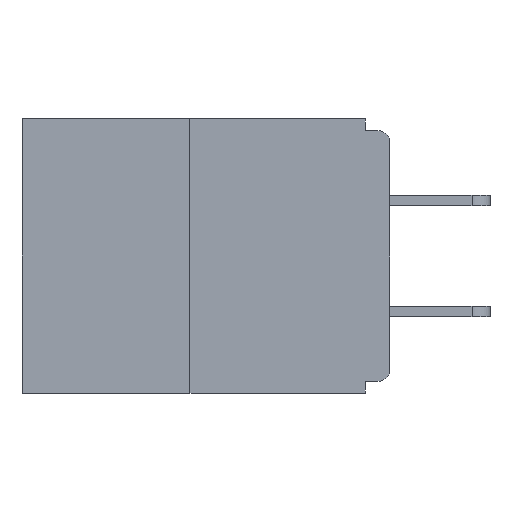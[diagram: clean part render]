
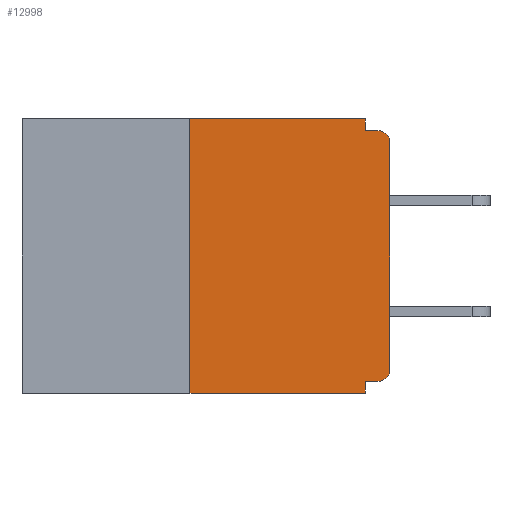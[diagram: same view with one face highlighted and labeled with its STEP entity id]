
A CAD part, left-side view. The second image highlights one B-rep face of the part: STEP entity #12998.
In plain terms, the highlighted planar face has unit normal (-1, 0, 0).
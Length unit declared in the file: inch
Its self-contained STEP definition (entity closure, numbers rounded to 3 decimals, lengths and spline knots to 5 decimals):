
#118 = DIRECTION ( 'NONE',  ( 0., 0., -1. ) ) ;
#300 = ORIENTED_EDGE ( 'NONE', *, *, #8440, .T. ) ;
#609 = VERTEX_POINT ( 'NONE', #5501 ) ;
#693 = CARTESIAN_POINT ( 'NONE',  ( 0., 0.015, -0.313 ) ) ;
#877 = DIRECTION ( 'NONE',  ( 0., -1., 0. ) ) ;
#916 = VECTOR ( 'NONE', #6796, 39.37008 ) ;
#1182 = DIRECTION ( 'NONE',  ( 0., 0., -1. ) ) ;
#2056 = LINE ( 'NONE', #11511, #4643 ) ;
#2653 = ORIENTED_EDGE ( 'NONE', *, *, #12278, .F. ) ;
#2808 = EDGE_CURVE ( 'NONE', #11994, #15550, #15641, .T. ) ;
#2951 = LINE ( 'NONE', #13225, #12132 ) ;
#3209 = CARTESIAN_POINT ( 'NONE',  ( 0., 0., -0.03 ) ) ;
#3536 = DIRECTION ( 'NONE',  ( 0., 0., 1. ) ) ;
#4190 = VERTEX_POINT ( 'NONE', #11120 ) ;
#4578 = EDGE_LOOP ( 'NONE', ( #9824, #7527, #5106, #11072, #5703, #300, #7327, #6595, #2653, #16163 ) ) ;
#4643 = VECTOR ( 'NONE', #1182, 39.37008 ) ;
#5106 = ORIENTED_EDGE ( 'NONE', *, *, #10989, .T. ) ;
#5346 = CARTESIAN_POINT ( 'NONE',  ( 0., 0., -0.015 ) ) ;
#5501 = CARTESIAN_POINT ( 'NONE',  ( 0., 0.015, -0.328 ) ) ;
#5656 = CARTESIAN_POINT ( 'NONE',  ( 0., 0.031, -0.328 ) ) ;
#5703 = ORIENTED_EDGE ( 'NONE', *, *, #7304, .F. ) ;
#5862 = CARTESIAN_POINT ( 'NONE',  ( 0., 0.031, -0.015 ) ) ;
#6021 = VERTEX_POINT ( 'NONE', #15294 ) ;
#6104 = VERTEX_POINT ( 'NONE', #5656 ) ;
#6595 = ORIENTED_EDGE ( 'NONE', *, *, #2808, .T. ) ;
#6708 = FACE_OUTER_BOUND ( 'NONE', #4578, .T. ) ;
#6796 = DIRECTION ( 'NONE',  ( 0., -1., 0. ) ) ;
#6824 = AXIS2_PLACEMENT_3D ( 'NONE', #693, #12034, #11977 ) ;
#6897 = CARTESIAN_POINT ( 'NONE',  ( 0., 0.015, -0.015 ) ) ;
#7217 = EDGE_CURVE ( 'NONE', #13805, #13820, #2056, .T. ) ;
#7221 = VECTOR ( 'NONE', #3536, 39.37008 ) ;
#7253 = CARTESIAN_POINT ( 'NONE',  ( 0., 0.46, 0. ) ) ;
#7304 = EDGE_CURVE ( 'NONE', #609, #6104, #11629, .T. ) ;
#7327 = ORIENTED_EDGE ( 'NONE', *, *, #16149, .T. ) ;
#7527 = ORIENTED_EDGE ( 'NONE', *, *, #11657, .F. ) ;
#7826 = VERTEX_POINT ( 'NONE', #14133 ) ;
#7867 = VECTOR ( 'NONE', #10351, 39.37008 ) ;
#8162 = LINE ( 'NONE', #11536, #14740 ) ;
#8440 = EDGE_CURVE ( 'NONE', #609, #4190, #14588, .T. ) ;
#9077 = CARTESIAN_POINT ( 'NONE',  ( 0., 0.015, -0.03 ) ) ;
#9128 = CARTESIAN_POINT ( 'NONE',  ( 0., 0., -0.328 ) ) ;
#9378 = LINE ( 'NONE', #7253, #15359 ) ;
#9507 = LINE ( 'NONE', #15644, #916 ) ;
#9747 = CARTESIAN_POINT ( 'NONE',  ( 0., 0.031, 0. ) ) ;
#9824 = ORIENTED_EDGE ( 'NONE', *, *, #9898, .F. ) ;
#9898 = EDGE_CURVE ( 'NONE', #14648, #13805, #9378, .T. ) ;
#10116 = VECTOR ( 'NONE', #14479, 39.37008 ) ;
#10157 = DIRECTION ( 'NONE',  ( 0., 0., 1. ) ) ;
#10245 = DIRECTION ( 'NONE',  ( -1., 0., 0. ) ) ;
#10293 = AXIS2_PLACEMENT_3D ( 'NONE', #9077, #10245, #118 ) ;
#10351 = DIRECTION ( 'NONE',  ( 0., 1., 0. ) ) ;
#10369 = EDGE_CURVE ( 'NONE', #6104, #7826, #2951, .T. ) ;
#10850 = DIRECTION ( 'NONE',  ( 0., 0., -1. ) ) ;
#10989 = EDGE_CURVE ( 'NONE', #6021, #7826, #9507, .T. ) ;
#11023 = CARTESIAN_POINT ( 'NONE',  ( 0., 0.46, 0. ) ) ;
#11072 = ORIENTED_EDGE ( 'NONE', *, *, #10369, .F. ) ;
#11120 = CARTESIAN_POINT ( 'NONE',  ( 0., 0., -0.313 ) ) ;
#11250 = CARTESIAN_POINT ( 'NONE',  ( 0., 0.25, 0. ) ) ;
#11511 = CARTESIAN_POINT ( 'NONE',  ( 0., 0.031, 0. ) ) ;
#11536 = CARTESIAN_POINT ( 'NONE',  ( 0., 0.25, 0. ) ) ;
#11629 = LINE ( 'NONE', #9128, #7867 ) ;
#11657 = EDGE_CURVE ( 'NONE', #6021, #14648, #8162, .T. ) ;
#11711 = CARTESIAN_POINT ( 'NONE',  ( 0., 0., 0. ) ) ;
#11714 = DIRECTION ( 'NONE',  ( 0., 0., -1. ) ) ;
#11977 = DIRECTION ( 'NONE',  ( 0., 0., -1. ) ) ;
#11994 = VERTEX_POINT ( 'NONE', #3209 ) ;
#12034 = DIRECTION ( 'NONE',  ( -1., 0., 0. ) ) ;
#12110 = LINE ( 'NONE', #5346, #10116 ) ;
#12132 = VECTOR ( 'NONE', #11714, 39.37008 ) ;
#12138 = PLANE ( 'NONE',  #12524 ) ;
#12194 = LINE ( 'NONE', #11711, #7221 ) ;
#12278 = EDGE_CURVE ( 'NONE', #13820, #15550, #12110, .T. ) ;
#12524 = AXIS2_PLACEMENT_3D ( 'NONE', #11023, #14713, #10850 ) ;
#12998 = ADVANCED_FACE ( 'NONE', ( #6708 ), #12138, .F. ) ;
#13225 = CARTESIAN_POINT ( 'NONE',  ( 0., 0.031, -0.343 ) ) ;
#13805 = VERTEX_POINT ( 'NONE', #9747 ) ;
#13820 = VERTEX_POINT ( 'NONE', #5862 ) ;
#14133 = CARTESIAN_POINT ( 'NONE',  ( 0., 0.031, -0.343 ) ) ;
#14479 = DIRECTION ( 'NONE',  ( 0., -1., 0. ) ) ;
#14588 = CIRCLE ( 'NONE', #6824, 0.015 ) ;
#14648 = VERTEX_POINT ( 'NONE', #11250 ) ;
#14713 = DIRECTION ( 'NONE',  ( 1., 0., 0. ) ) ;
#14740 = VECTOR ( 'NONE', #10157, 39.37008 ) ;
#15294 = CARTESIAN_POINT ( 'NONE',  ( 0., 0.25, -0.343 ) ) ;
#15359 = VECTOR ( 'NONE', #877, 39.37008 ) ;
#15550 = VERTEX_POINT ( 'NONE', #6897 ) ;
#15641 = CIRCLE ( 'NONE', #10293, 0.015 ) ;
#15644 = CARTESIAN_POINT ( 'NONE',  ( 0., 0.46, -0.343 ) ) ;
#16149 = EDGE_CURVE ( 'NONE', #4190, #11994, #12194, .T. ) ;
#16163 = ORIENTED_EDGE ( 'NONE', *, *, #7217, .F. ) ;
